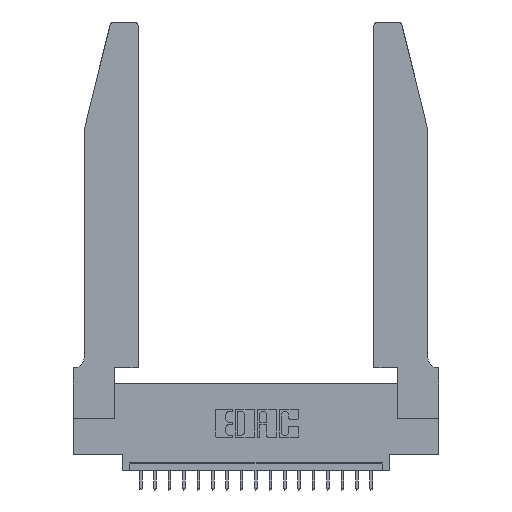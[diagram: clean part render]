
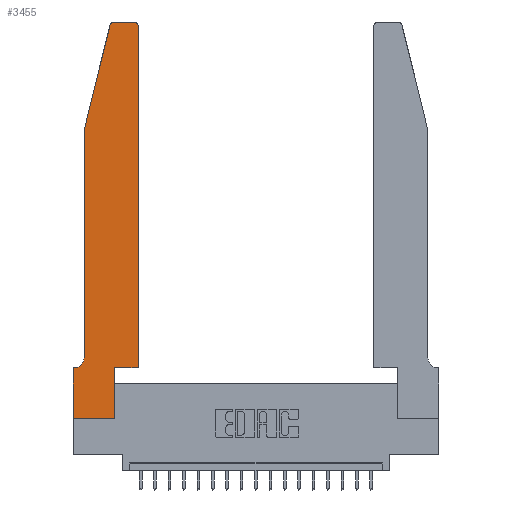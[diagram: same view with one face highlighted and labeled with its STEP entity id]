
A CAD part, top view. The second image highlights one B-rep face of the part: STEP entity #3455.
In plain terms, the highlighted planar face has unit normal (0, 0, 1).
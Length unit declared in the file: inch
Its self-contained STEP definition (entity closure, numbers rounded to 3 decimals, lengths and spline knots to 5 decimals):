
#272 = DIRECTION ( 'NONE',  ( 0., 1., 0. ) ) ;
#349 = LINE ( 'NONE', #556, #15875 ) ;
#396 = CARTESIAN_POINT ( 'NONE',  ( 0.0055, 0.35, 0.37 ) ) ;
#517 = EDGE_CURVE ( 'NONE', #5721, #16268, #7379, .T. ) ;
#556 = CARTESIAN_POINT ( 'NONE',  ( 0., 0., 0.37 ) ) ;
#630 = DIRECTION ( 'NONE',  ( 0., 0., 1. ) ) ;
#729 = DIRECTION ( 'NONE',  ( 0., -1., 0. ) ) ;
#893 = DIRECTION ( 'NONE',  ( -1., 0., 0. ) ) ;
#958 = DIRECTION ( 'NONE',  ( 1., 0., 0. ) ) ;
#1084 = ORIENTED_EDGE ( 'NONE', *, *, #18626, .T. ) ;
#2272 = AXIS2_PLACEMENT_3D ( 'NONE', #5293, #18447, #958 ) ;
#2486 = EDGE_CURVE ( 'NONE', #4015, #15714, #10018, .T. ) ;
#2522 = ORIENTED_EDGE ( 'NONE', *, *, #5058, .T. ) ;
#2537 = DIRECTION ( 'NONE',  ( 0., 0., 1. ) ) ;
#2608 = EDGE_CURVE ( 'NONE', #19921, #19587, #4101, .T. ) ;
#2673 = CARTESIAN_POINT ( 'NONE',  ( 0.0755, 0.35, 0.37 ) ) ;
#3072 = CARTESIAN_POINT ( 'NONE',  ( 0.0755, 2., 0.37 ) ) ;
#3176 = DIRECTION ( 'NONE',  ( -0.239, -0.971, 0. ) ) ;
#3455 = ADVANCED_FACE ( 'NONE', ( #5577 ), #13266, .T. ) ;
#3521 = CARTESIAN_POINT ( 'NONE',  ( 0.4505, 0.35, 0.37 ) ) ;
#3546 = ORIENTED_EDGE ( 'NONE', *, *, #20711, .T. ) ;
#3802 = VERTEX_POINT ( 'NONE', #6615 ) ;
#4015 = VERTEX_POINT ( 'NONE', #20599 ) ;
#4056 = ORIENTED_EDGE ( 'NONE', *, *, #2608, .T. ) ;
#4101 = LINE ( 'NONE', #15230, #15003 ) ;
#4655 = DIRECTION ( 'NONE',  ( -1., 0., 0. ) ) ;
#4689 = CARTESIAN_POINT ( 'NONE',  ( 0., 0.35, 0.37 ) ) ;
#4723 = CARTESIAN_POINT ( 'NONE',  ( 0.2865, 0., 0.37 ) ) ;
#4728 = VECTOR ( 'NONE', #5248, 39.37008 ) ;
#4754 = DIRECTION ( 'NONE',  ( 0., 0., -1. ) ) ;
#5058 = EDGE_CURVE ( 'NONE', #7305, #10185, #11504, .T. ) ;
#5195 = CARTESIAN_POINT ( 'NONE',  ( 0.4505, 0.35, 0.37 ) ) ;
#5248 = DIRECTION ( 'NONE',  ( 1., 0., 0. ) ) ;
#5254 = ORIENTED_EDGE ( 'NONE', *, *, #13766, .T. ) ;
#5293 = CARTESIAN_POINT ( 'NONE',  ( 0.284, 2.72, 0.37 ) ) ;
#5530 = EDGE_CURVE ( 'NONE', #15714, #11903, #14477, .T. ) ;
#5577 = FACE_OUTER_BOUND ( 'NONE', #14049, .T. ) ;
#5692 = ORIENTED_EDGE ( 'NONE', *, *, #17388, .T. ) ;
#5721 = VERTEX_POINT ( 'NONE', #4689 ) ;
#6058 = CARTESIAN_POINT ( 'NONE',  ( 0., 0., 0.37 ) ) ;
#6301 = AXIS2_PLACEMENT_3D ( 'NONE', #15167, #2537, #13773 ) ;
#6615 = CARTESIAN_POINT ( 'NONE',  ( 0.2865, 0.35, 0.37 ) ) ;
#6895 = VECTOR ( 'NONE', #12419, 39.37008 ) ;
#6977 = ORIENTED_EDGE ( 'NONE', *, *, #517, .T. ) ;
#7056 = DIRECTION ( 'NONE',  ( 0., 1., 0. ) ) ;
#7305 = VERTEX_POINT ( 'NONE', #11400 ) ;
#7379 = LINE ( 'NONE', #15276, #10569 ) ;
#7506 = ORIENTED_EDGE ( 'NONE', *, *, #15345, .T. ) ;
#7760 = CARTESIAN_POINT ( 'NONE',  ( 0.0055, 0.42, 0.37 ) ) ;
#7926 = LINE ( 'NONE', #2673, #6895 ) ;
#8119 = VERTEX_POINT ( 'NONE', #4723 ) ;
#8884 = CARTESIAN_POINT ( 'NONE',  ( 0., 0.35, 0.37 ) ) ;
#9624 = ORIENTED_EDGE ( 'NONE', *, *, #5530, .T. ) ;
#9669 = CARTESIAN_POINT ( 'NONE',  ( 0.4505, 2.72, 0.37 ) ) ;
#9890 = VECTOR ( 'NONE', #272, 39.37008 ) ;
#10018 = LINE ( 'NONE', #5195, #9890 ) ;
#10185 = VERTEX_POINT ( 'NONE', #10205 ) ;
#10205 = CARTESIAN_POINT ( 'NONE',  ( 0.25487, 2.72718, 0.37 ) ) ;
#10285 = DIRECTION ( 'NONE',  ( 1., 0., 0. ) ) ;
#10569 = VECTOR ( 'NONE', #729, 39.37008 ) ;
#11184 = EDGE_CURVE ( 'NONE', #19587, #17824, #11387, .T. ) ;
#11387 = CIRCLE ( 'NONE', #18225, 0.07 ) ;
#11400 = CARTESIAN_POINT ( 'NONE',  ( 0.284, 2.75, 0.37 ) ) ;
#11504 = CIRCLE ( 'NONE', #2272, 0.03 ) ;
#11903 = VERTEX_POINT ( 'NONE', #11995 ) ;
#11995 = CARTESIAN_POINT ( 'NONE',  ( 0.4205, 2.75, 0.37 ) ) ;
#12083 = LINE ( 'NONE', #13466, #19707 ) ;
#12419 = DIRECTION ( 'NONE',  ( -1., 0., 0. ) ) ;
#12606 = LINE ( 'NONE', #3072, #16924 ) ;
#12688 = ORIENTED_EDGE ( 'NONE', *, *, #14694, .T. ) ;
#13266 = PLANE ( 'NONE',  #14604 ) ;
#13398 = DIRECTION ( 'NONE',  ( 1., 0., 0. ) ) ;
#13466 = CARTESIAN_POINT ( 'NONE',  ( 0.2865, 0.35, 0.37 ) ) ;
#13497 = VECTOR ( 'NONE', #893, 39.37008 ) ;
#13766 = EDGE_CURVE ( 'NONE', #10185, #19921, #12606, .T. ) ;
#13773 = DIRECTION ( 'NONE',  ( 1., 0., 0. ) ) ;
#14049 = EDGE_LOOP ( 'NONE', ( #7506, #2522, #5254, #4056, #14515, #3546, #6977, #12688, #5692, #1084, #18658, #9624 ) ) ;
#14408 = CARTESIAN_POINT ( 'NONE',  ( 0.0755, 2., 0.37 ) ) ;
#14477 = CIRCLE ( 'NONE', #6301, 0.03 ) ;
#14515 = ORIENTED_EDGE ( 'NONE', *, *, #11184, .T. ) ;
#14604 = AXIS2_PLACEMENT_3D ( 'NONE', #8884, #630, #10285 ) ;
#14694 = EDGE_CURVE ( 'NONE', #16268, #8119, #349, .T. ) ;
#15003 = VECTOR ( 'NONE', #17043, 39.37008 ) ;
#15167 = CARTESIAN_POINT ( 'NONE',  ( 0.4205, 2.72, 0.37 ) ) ;
#15230 = CARTESIAN_POINT ( 'NONE',  ( 0.0755, 2., 0.37 ) ) ;
#15276 = CARTESIAN_POINT ( 'NONE',  ( 0., 0., 0.37 ) ) ;
#15345 = EDGE_CURVE ( 'NONE', #11903, #7305, #20153, .T. ) ;
#15714 = VERTEX_POINT ( 'NONE', #9669 ) ;
#15761 = CARTESIAN_POINT ( 'NONE',  ( 0.0755, 0.42, 0.37 ) ) ;
#15875 = VECTOR ( 'NONE', #13398, 39.37008 ) ;
#16268 = VERTEX_POINT ( 'NONE', #6058 ) ;
#16785 = LINE ( 'NONE', #3521, #4728 ) ;
#16924 = VECTOR ( 'NONE', #3176, 39.37008 ) ;
#17043 = DIRECTION ( 'NONE',  ( 0., -1., 0. ) ) ;
#17388 = EDGE_CURVE ( 'NONE', #8119, #3802, #12083, .T. ) ;
#17824 = VERTEX_POINT ( 'NONE', #396 ) ;
#18225 = AXIS2_PLACEMENT_3D ( 'NONE', #7760, #4754, #4655 ) ;
#18447 = DIRECTION ( 'NONE',  ( 0., 0., 1. ) ) ;
#18626 = EDGE_CURVE ( 'NONE', #3802, #4015, #16785, .T. ) ;
#18658 = ORIENTED_EDGE ( 'NONE', *, *, #2486, .T. ) ;
#19587 = VERTEX_POINT ( 'NONE', #15761 ) ;
#19707 = VECTOR ( 'NONE', #7056, 39.37008 ) ;
#19921 = VERTEX_POINT ( 'NONE', #14408 ) ;
#20049 = CARTESIAN_POINT ( 'NONE',  ( 0.2605, 2.75, 0.37 ) ) ;
#20153 = LINE ( 'NONE', #20049, #13497 ) ;
#20599 = CARTESIAN_POINT ( 'NONE',  ( 0.4505, 0.35, 0.37 ) ) ;
#20711 = EDGE_CURVE ( 'NONE', #17824, #5721, #7926, .T. ) ;
